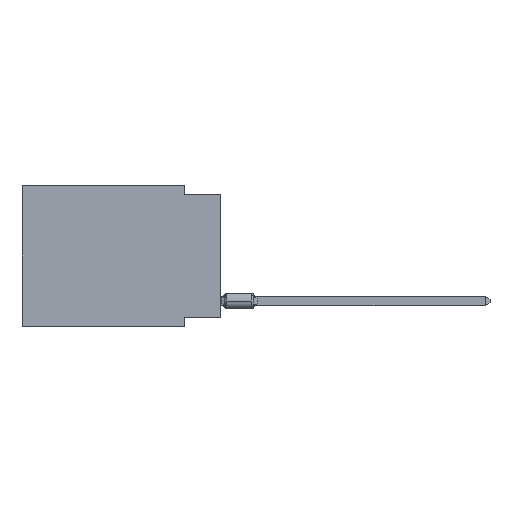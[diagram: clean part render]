
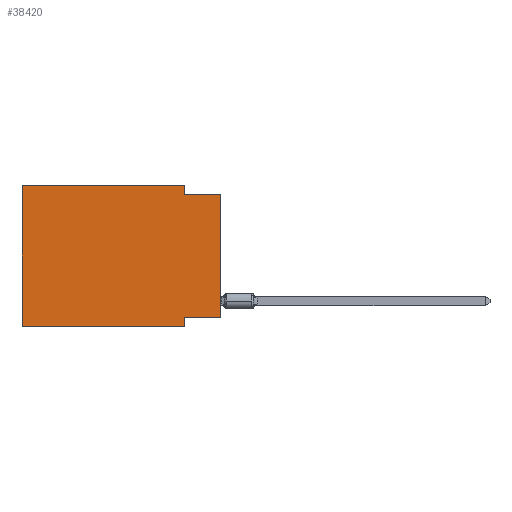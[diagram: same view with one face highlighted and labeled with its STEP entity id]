
A CAD part, left-side view. The second image highlights one B-rep face of the part: STEP entity #38420.
In plain terms, the highlighted planar face has unit normal (-1, 0, 0).
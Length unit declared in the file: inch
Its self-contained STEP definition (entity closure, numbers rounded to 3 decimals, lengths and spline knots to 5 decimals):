
#1527 = CARTESIAN_POINT ( 'NONE',  ( 0., 0., -0.025 ) ) ;
#1617 = VERTEX_POINT ( 'NONE', #19780 ) ;
#2235 = LINE ( 'NONE', #48298, #6067 ) ;
#2337 = DIRECTION ( 'NONE',  ( 0., -1., 0. ) ) ;
#2573 = LINE ( 'NONE', #48894, #5926 ) ;
#2585 = LINE ( 'NONE', #44884, #30508 ) ;
#2639 = CARTESIAN_POINT ( 'NONE',  ( 0., 0.55, 0. ) ) ;
#3137 = DIRECTION ( 'NONE',  ( 0., 0., -1. ) ) ;
#3818 = EDGE_LOOP ( 'NONE', ( #19152, #22197, #9410, #23767, #16048, #28719, #10551, #18249 ) ) ;
#5320 = VERTEX_POINT ( 'NONE', #45209 ) ;
#5926 = VECTOR ( 'NONE', #14420, 39.37008 ) ;
#6067 = VECTOR ( 'NONE', #13576, 39.37008 ) ;
#7879 = CARTESIAN_POINT ( 'NONE',  ( 0., 0.55, 0. ) ) ;
#9410 = ORIENTED_EDGE ( 'NONE', *, *, #9448, .F. ) ;
#9448 = EDGE_CURVE ( 'NONE', #38834, #1617, #28979, .T. ) ;
#10551 = ORIENTED_EDGE ( 'NONE', *, *, #46356, .F. ) ;
#11533 = DIRECTION ( 'NONE',  ( 0., -1., 0. ) ) ;
#13125 = EDGE_CURVE ( 'NONE', #14947, #38834, #2235, .T. ) ;
#13330 = EDGE_CURVE ( 'NONE', #16805, #5320, #29650, .T. ) ;
#13576 = DIRECTION ( 'NONE',  ( 0., -1., 0. ) ) ;
#14096 = CARTESIAN_POINT ( 'NONE',  ( 0., 0., -0.365 ) ) ;
#14420 = DIRECTION ( 'NONE',  ( 0., 0., -1. ) ) ;
#14790 = VERTEX_POINT ( 'NONE', #1527 ) ;
#14947 = VERTEX_POINT ( 'NONE', #45334 ) ;
#15664 = CARTESIAN_POINT ( 'NONE',  ( 0., 0.1, -0.365 ) ) ;
#16048 = ORIENTED_EDGE ( 'NONE', *, *, #33390, .F. ) ;
#16805 = VERTEX_POINT ( 'NONE', #30181 ) ;
#17639 = VECTOR ( 'NONE', #19459, 39.37008 ) ;
#17922 = CARTESIAN_POINT ( 'NONE',  ( 0., 0.1, 0. ) ) ;
#18249 = ORIENTED_EDGE ( 'NONE', *, *, #41473, .F. ) ;
#18496 = FACE_OUTER_BOUND ( 'NONE', #3818, .T. ) ;
#19152 = ORIENTED_EDGE ( 'NONE', *, *, #33298, .T. ) ;
#19459 = DIRECTION ( 'NONE',  ( 0., 0., 1. ) ) ;
#19722 = LINE ( 'NONE', #34310, #24030 ) ;
#19780 = CARTESIAN_POINT ( 'NONE',  ( 0., 0.1, -0.025 ) ) ;
#21669 = CARTESIAN_POINT ( 'NONE',  ( 0., 0., -0.365 ) ) ;
#22197 = ORIENTED_EDGE ( 'NONE', *, *, #39732, .F. ) ;
#23767 = ORIENTED_EDGE ( 'NONE', *, *, #13125, .F. ) ;
#24030 = VECTOR ( 'NONE', #34555, 39.37008 ) ;
#25235 = DIRECTION ( 'NONE',  ( 0., 0., -1. ) ) ;
#25450 = LINE ( 'NONE', #21669, #41106 ) ;
#25543 = VERTEX_POINT ( 'NONE', #15664 ) ;
#26048 = PLANE ( 'NONE',  #34463 ) ;
#28719 = ORIENTED_EDGE ( 'NONE', *, *, #13330, .T. ) ;
#28979 = LINE ( 'NONE', #17922, #31517 ) ;
#29650 = LINE ( 'NONE', #41505, #49523 ) ;
#30181 = CARTESIAN_POINT ( 'NONE',  ( 0., 0.55, -0.39 ) ) ;
#30508 = VECTOR ( 'NONE', #2337, 39.37008 ) ;
#31030 = VERTEX_POINT ( 'NONE', #14096 ) ;
#31517 = VECTOR ( 'NONE', #25235, 39.37008 ) ;
#33298 = EDGE_CURVE ( 'NONE', #31030, #14790, #19722, .T. ) ;
#33390 = EDGE_CURVE ( 'NONE', #16805, #14947, #42374, .T. ) ;
#34310 = CARTESIAN_POINT ( 'NONE',  ( 0., 0., 0. ) ) ;
#34463 = AXIS2_PLACEMENT_3D ( 'NONE', #2639, #37634, #3137 ) ;
#34555 = DIRECTION ( 'NONE',  ( 0., 0., 1. ) ) ;
#37634 = DIRECTION ( 'NONE',  ( 1., 0., 0. ) ) ;
#38420 = ADVANCED_FACE ( 'NONE', ( #18496 ), #26048, .F. ) ;
#38834 = VERTEX_POINT ( 'NONE', #39963 ) ;
#39732 = EDGE_CURVE ( 'NONE', #1617, #14790, #2585, .T. ) ;
#39963 = CARTESIAN_POINT ( 'NONE',  ( 0., 0.1, 0. ) ) ;
#41106 = VECTOR ( 'NONE', #46072, 39.37008 ) ;
#41473 = EDGE_CURVE ( 'NONE', #31030, #25543, #25450, .T. ) ;
#41505 = CARTESIAN_POINT ( 'NONE',  ( 0., 0.55, -0.39 ) ) ;
#42374 = LINE ( 'NONE', #7879, #17639 ) ;
#44884 = CARTESIAN_POINT ( 'NONE',  ( 0., 0., -0.025 ) ) ;
#45209 = CARTESIAN_POINT ( 'NONE',  ( 0., 0.1, -0.39 ) ) ;
#45334 = CARTESIAN_POINT ( 'NONE',  ( 0., 0.55, 0. ) ) ;
#46072 = DIRECTION ( 'NONE',  ( 0., 1., 0. ) ) ;
#46356 = EDGE_CURVE ( 'NONE', #25543, #5320, #2573, .T. ) ;
#48298 = CARTESIAN_POINT ( 'NONE',  ( 0., 0.55, 0. ) ) ;
#48894 = CARTESIAN_POINT ( 'NONE',  ( 0., 0.1, -0.39 ) ) ;
#49523 = VECTOR ( 'NONE', #11533, 39.37008 ) ;
